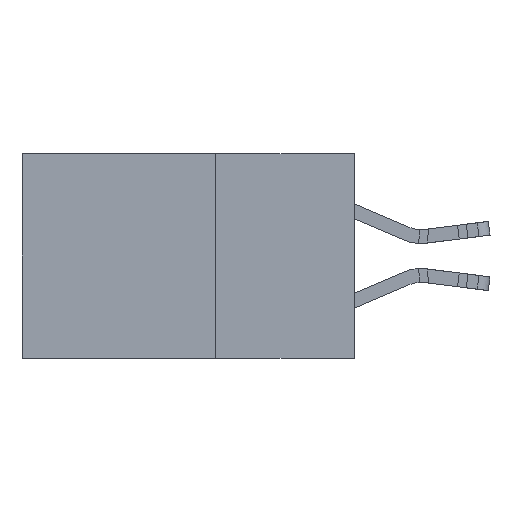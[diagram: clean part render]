
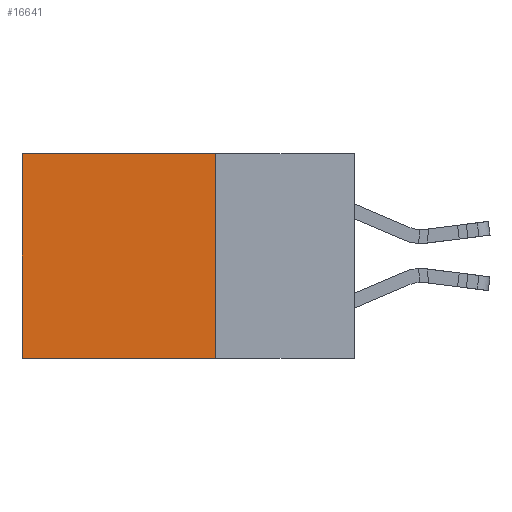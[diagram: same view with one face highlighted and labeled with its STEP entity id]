
A CAD part, left-side view. The second image highlights one B-rep face of the part: STEP entity #16641.
In plain terms, the highlighted planar face has unit normal (-1, 0, 0).
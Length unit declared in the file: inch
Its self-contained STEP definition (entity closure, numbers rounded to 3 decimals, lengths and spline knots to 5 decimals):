
#527 = ORIENTED_EDGE ( 'NONE', *, *, #7285, .F. ) ;
#866 = CARTESIAN_POINT ( 'NONE',  ( 0.298, 0.6, 0. ) ) ;
#967 = DIRECTION ( 'NONE',  ( 0., 1., 0. ) ) ;
#3654 = CARTESIAN_POINT ( 'NONE',  ( 0.298, 0.25, -0.37 ) ) ;
#4186 = VERTEX_POINT ( 'NONE', #5870 ) ;
#4493 = CARTESIAN_POINT ( 'NONE',  ( 0.298, 0.25, 0. ) ) ;
#5870 = CARTESIAN_POINT ( 'NONE',  ( 0.298, 0.6, -0.37 ) ) ;
#5878 = VECTOR ( 'NONE', #17085, 39.37008 ) ;
#6364 = VECTOR ( 'NONE', #8442, 39.37008 ) ;
#6585 = VERTEX_POINT ( 'NONE', #26139 ) ;
#6853 = DIRECTION ( 'NONE',  ( 0., 0., -1. ) ) ;
#7285 = EDGE_CURVE ( 'NONE', #15192, #4186, #11367, .T. ) ;
#8442 = DIRECTION ( 'NONE',  ( 0., 0., -1. ) ) ;
#9317 = VECTOR ( 'NONE', #967, 39.37008 ) ;
#10323 = EDGE_CURVE ( 'NONE', #6585, #19190, #21692, .T. ) ;
#10543 = EDGE_CURVE ( 'NONE', #19190, #4186, #22040, .T. ) ;
#11367 = LINE ( 'NONE', #28534, #5878 ) ;
#13107 = EDGE_LOOP ( 'NONE', ( #22164, #527, #25150, #13319 ) ) ;
#13228 = AXIS2_PLACEMENT_3D ( 'NONE', #4493, #20811, #6853 ) ;
#13319 = ORIENTED_EDGE ( 'NONE', *, *, #10323, .T. ) ;
#15192 = VERTEX_POINT ( 'NONE', #3654 ) ;
#16142 = PLANE ( 'NONE',  #13228 ) ;
#16546 = LINE ( 'NONE', #22388, #6364 ) ;
#16641 = ADVANCED_FACE ( 'NONE', ( #21419 ), #16142, .F. ) ;
#17085 = DIRECTION ( 'NONE',  ( 0., 1., 0. ) ) ;
#18098 = CARTESIAN_POINT ( 'NONE',  ( 0.298, 0.6, 0. ) ) ;
#19190 = VERTEX_POINT ( 'NONE', #866 ) ;
#20811 = DIRECTION ( 'NONE',  ( 1., 0., 0. ) ) ;
#21419 = FACE_OUTER_BOUND ( 'NONE', #13107, .T. ) ;
#21692 = LINE ( 'NONE', #28813, #9317 ) ;
#22040 = LINE ( 'NONE', #18098, #27463 ) ;
#22164 = ORIENTED_EDGE ( 'NONE', *, *, #10543, .T. ) ;
#22388 = CARTESIAN_POINT ( 'NONE',  ( 0.298, 0.25, 0. ) ) ;
#22802 = DIRECTION ( 'NONE',  ( 0., 0., -1. ) ) ;
#24257 = EDGE_CURVE ( 'NONE', #6585, #15192, #16546, .T. ) ;
#25150 = ORIENTED_EDGE ( 'NONE', *, *, #24257, .F. ) ;
#26139 = CARTESIAN_POINT ( 'NONE',  ( 0.298, 0.25, 0. ) ) ;
#27463 = VECTOR ( 'NONE', #22802, 39.37008 ) ;
#28534 = CARTESIAN_POINT ( 'NONE',  ( 0.298, 0.25, -0.37 ) ) ;
#28813 = CARTESIAN_POINT ( 'NONE',  ( 0.298, 0.25, 0. ) ) ;
